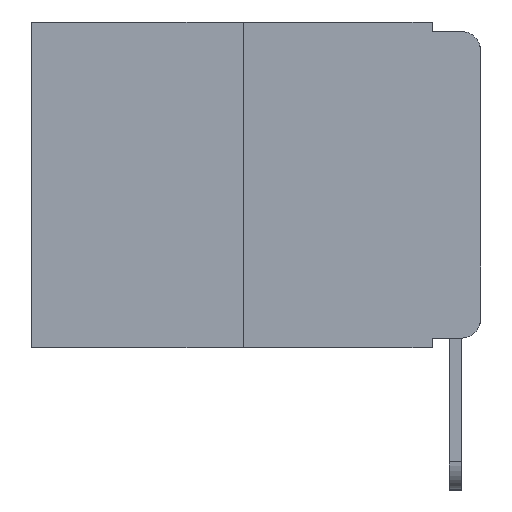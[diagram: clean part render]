
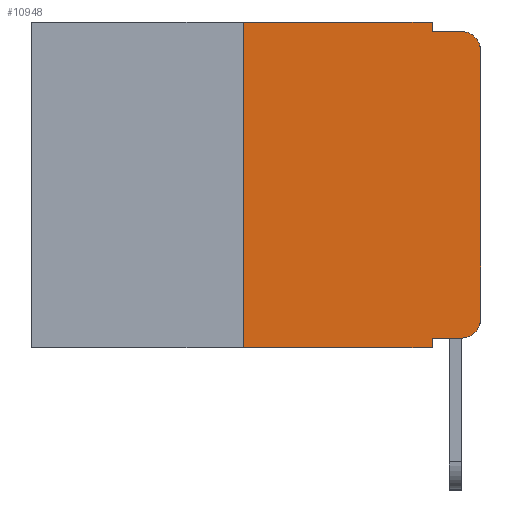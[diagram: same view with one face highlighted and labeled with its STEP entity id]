
A CAD part, left-side view. The second image highlights one B-rep face of the part: STEP entity #10948.
In plain terms, the highlighted planar face has unit normal (-1, 0, 0).
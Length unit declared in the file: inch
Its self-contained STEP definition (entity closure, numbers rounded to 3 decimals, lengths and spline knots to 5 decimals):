
#394 = CIRCLE ( 'NONE', #14814, 0.02 ) ;
#479 = CARTESIAN_POINT ( 'NONE',  ( 0., 0.02, -0.03 ) ) ;
#806 = DIRECTION ( 'NONE',  ( 0., 0., 1. ) ) ;
#2377 = EDGE_CURVE ( 'NONE', #5211, #4928, #6977, .T. ) ;
#3000 = ORIENTED_EDGE ( 'NONE', *, *, #13985, .T. ) ;
#3097 = DIRECTION ( 'NONE',  ( 0., 0., 1. ) ) ;
#3484 = CARTESIAN_POINT ( 'NONE',  ( 0., 0.473, -0.343 ) ) ;
#3791 = VECTOR ( 'NONE', #806, 39.37008 ) ;
#4471 = DIRECTION ( 'NONE',  ( 0., 0., -1. ) ) ;
#4791 = ORIENTED_EDGE ( 'NONE', *, *, #13275, .F. ) ;
#4820 = CIRCLE ( 'NONE', #7539, 0.02 ) ;
#4900 = LINE ( 'NONE', #3484, #5739 ) ;
#4914 = CARTESIAN_POINT ( 'NONE',  ( 0., 0.051, 0. ) ) ;
#4928 = VERTEX_POINT ( 'NONE', #13803 ) ;
#5211 = VERTEX_POINT ( 'NONE', #15947 ) ;
#5404 = CARTESIAN_POINT ( 'NONE',  ( 0., 0.25, -0.343 ) ) ;
#5689 = VERTEX_POINT ( 'NONE', #7434 ) ;
#5739 = VECTOR ( 'NONE', #10406, 39.37008 ) ;
#5939 = CARTESIAN_POINT ( 'NONE',  ( 0., 0.051, 0. ) ) ;
#5944 = EDGE_CURVE ( 'NONE', #12716, #5689, #15645, .T. ) ;
#5990 = DIRECTION ( 'NONE',  ( 0., -1., 0. ) ) ;
#6395 = ORIENTED_EDGE ( 'NONE', *, *, #15223, .T. ) ;
#6422 = LINE ( 'NONE', #17519, #14662 ) ;
#6513 = CARTESIAN_POINT ( 'NONE',  ( 0., 0.02, -0.333 ) ) ;
#6588 = LINE ( 'NONE', #11354, #15943 ) ;
#6977 = LINE ( 'NONE', #13020, #3791 ) ;
#7085 = CARTESIAN_POINT ( 'NONE',  ( 0., 0.051, 0. ) ) ;
#7393 = DIRECTION ( 'NONE',  ( 0., -1., 0. ) ) ;
#7434 = CARTESIAN_POINT ( 'NONE',  ( 0., 0.051, -0.01 ) ) ;
#7539 = AXIS2_PLACEMENT_3D ( 'NONE', #479, #10025, #14182 ) ;
#7540 = FACE_OUTER_BOUND ( 'NONE', #8451, .T. ) ;
#7570 = VECTOR ( 'NONE', #5990, 39.37008 ) ;
#7974 = VECTOR ( 'NONE', #14382, 39.37008 ) ;
#7986 = VECTOR ( 'NONE', #3097, 39.37008 ) ;
#8253 = VERTEX_POINT ( 'NONE', #13002 ) ;
#8421 = LINE ( 'NONE', #12779, #7986 ) ;
#8451 = EDGE_LOOP ( 'NONE', ( #17596, #16530, #9064, #16156, #4791, #9293, #13183, #10477, #3000, #6395 ) ) ;
#8631 = EDGE_CURVE ( 'NONE', #10981, #8253, #10358, .T. ) ;
#8697 = PLANE ( 'NONE',  #9069 ) ;
#9064 = ORIENTED_EDGE ( 'NONE', *, *, #15967, .F. ) ;
#9069 = AXIS2_PLACEMENT_3D ( 'NONE', #9931, #11341, #13972 ) ;
#9293 = ORIENTED_EDGE ( 'NONE', *, *, #9322, .F. ) ;
#9322 = EDGE_CURVE ( 'NONE', #9814, #15034, #8421, .T. ) ;
#9513 = VECTOR ( 'NONE', #16744, 39.37008 ) ;
#9814 = VERTEX_POINT ( 'NONE', #5404 ) ;
#9931 = CARTESIAN_POINT ( 'NONE',  ( 0., 0.473, 0. ) ) ;
#10025 = DIRECTION ( 'NONE',  ( -1., 0., 0. ) ) ;
#10358 = LINE ( 'NONE', #5939, #9513 ) ;
#10406 = DIRECTION ( 'NONE',  ( 0., -1., 0. ) ) ;
#10477 = ORIENTED_EDGE ( 'NONE', *, *, #8631, .F. ) ;
#10720 = CARTESIAN_POINT ( 'NONE',  ( 0., 0.25, 0. ) ) ;
#10948 = ADVANCED_FACE ( 'NONE', ( #7540 ), #8697, .F. ) ;
#10981 = VERTEX_POINT ( 'NONE', #11416 ) ;
#11172 = LINE ( 'NONE', #11239, #7570 ) ;
#11239 = CARTESIAN_POINT ( 'NONE',  ( 0., 0.051, -0.01 ) ) ;
#11341 = DIRECTION ( 'NONE',  ( 1., 0., 0. ) ) ;
#11354 = CARTESIAN_POINT ( 'NONE',  ( 0., 0.051, -0.333 ) ) ;
#11375 = CARTESIAN_POINT ( 'NONE',  ( 0., 0.02, -0.313 ) ) ;
#11416 = CARTESIAN_POINT ( 'NONE',  ( 0., 0.051, -0.333 ) ) ;
#11664 = CARTESIAN_POINT ( 'NONE',  ( 0., 0.02, -0.01 ) ) ;
#12716 = VERTEX_POINT ( 'NONE', #7085 ) ;
#12779 = CARTESIAN_POINT ( 'NONE',  ( 0., 0.25, 0. ) ) ;
#12903 = VERTEX_POINT ( 'NONE', #11664 ) ;
#13002 = CARTESIAN_POINT ( 'NONE',  ( 0., 0.051, -0.343 ) ) ;
#13020 = CARTESIAN_POINT ( 'NONE',  ( 0., 0., 0. ) ) ;
#13183 = ORIENTED_EDGE ( 'NONE', *, *, #14125, .T. ) ;
#13275 = EDGE_CURVE ( 'NONE', #15034, #12716, #6422, .T. ) ;
#13803 = CARTESIAN_POINT ( 'NONE',  ( 0., 0., -0.03 ) ) ;
#13972 = DIRECTION ( 'NONE',  ( 0., 0., -1. ) ) ;
#13985 = EDGE_CURVE ( 'NONE', #10981, #16850, #6588, .T. ) ;
#14054 = DIRECTION ( 'NONE',  ( -1., 0., 0. ) ) ;
#14125 = EDGE_CURVE ( 'NONE', #9814, #8253, #4900, .T. ) ;
#14182 = DIRECTION ( 'NONE',  ( 0., 0., -1. ) ) ;
#14382 = DIRECTION ( 'NONE',  ( 0., 0., -1. ) ) ;
#14662 = VECTOR ( 'NONE', #16204, 39.37008 ) ;
#14814 = AXIS2_PLACEMENT_3D ( 'NONE', #11375, #14054, #4471 ) ;
#15034 = VERTEX_POINT ( 'NONE', #10720 ) ;
#15223 = EDGE_CURVE ( 'NONE', #16850, #5211, #394, .T. ) ;
#15645 = LINE ( 'NONE', #4914, #7974 ) ;
#15943 = VECTOR ( 'NONE', #7393, 39.37008 ) ;
#15947 = CARTESIAN_POINT ( 'NONE',  ( 0., 0., -0.313 ) ) ;
#15967 = EDGE_CURVE ( 'NONE', #5689, #12903, #11172, .T. ) ;
#16142 = EDGE_CURVE ( 'NONE', #4928, #12903, #4820, .T. ) ;
#16156 = ORIENTED_EDGE ( 'NONE', *, *, #5944, .F. ) ;
#16204 = DIRECTION ( 'NONE',  ( 0., -1., 0. ) ) ;
#16530 = ORIENTED_EDGE ( 'NONE', *, *, #16142, .T. ) ;
#16744 = DIRECTION ( 'NONE',  ( 0., 0., -1. ) ) ;
#16850 = VERTEX_POINT ( 'NONE', #6513 ) ;
#17519 = CARTESIAN_POINT ( 'NONE',  ( 0., 0.473, 0. ) ) ;
#17596 = ORIENTED_EDGE ( 'NONE', *, *, #2377, .T. ) ;
